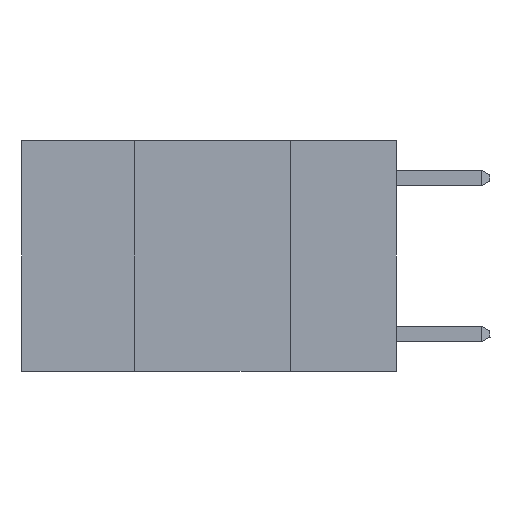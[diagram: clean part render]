
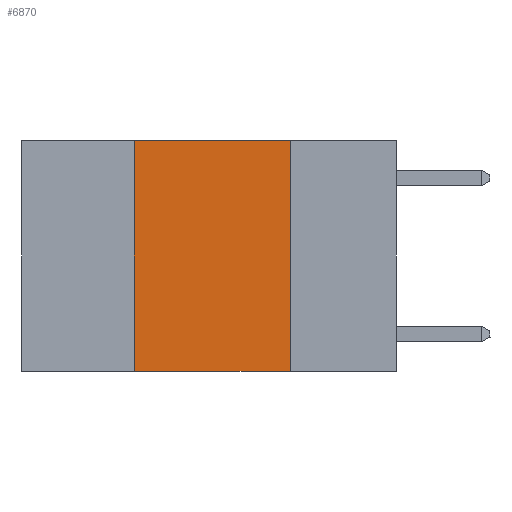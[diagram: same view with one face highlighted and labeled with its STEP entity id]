
A CAD part, left-side view. The second image highlights one B-rep face of the part: STEP entity #6870.
In plain terms, the highlighted planar face has unit normal (-1, 0, 0).
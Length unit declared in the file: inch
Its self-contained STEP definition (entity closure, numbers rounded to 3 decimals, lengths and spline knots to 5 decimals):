
#590 = EDGE_LOOP ( 'NONE', ( #928, #8907, #14900, #12111 ) ) ;
#600 = CARTESIAN_POINT ( 'NONE',  ( 0., 0.42, 0. ) ) ;
#683 = CARTESIAN_POINT ( 'NONE',  ( 0., 0.42, -0.37 ) ) ;
#928 = ORIENTED_EDGE ( 'NONE', *, *, #16280, .F. ) ;
#1712 = LINE ( 'NONE', #1965, #7684 ) ;
#1965 = CARTESIAN_POINT ( 'NONE',  ( 0., 0.17, 0. ) ) ;
#3017 = VECTOR ( 'NONE', #3855, 39.37008 ) ;
#3074 = VECTOR ( 'NONE', #6074, 39.37008 ) ;
#3231 = DIRECTION ( 'NONE',  ( 0., 0., -1. ) ) ;
#3290 = EDGE_CURVE ( 'NONE', #13494, #14641, #10229, .T. ) ;
#3325 = LINE ( 'NONE', #4605, #8217 ) ;
#3855 = DIRECTION ( 'NONE',  ( 0., -1., 0. ) ) ;
#4101 = VERTEX_POINT ( 'NONE', #16416 ) ;
#4605 = CARTESIAN_POINT ( 'NONE',  ( 0., 0.6, -0.37 ) ) ;
#5047 = CARTESIAN_POINT ( 'NONE',  ( 0., 0.6, 0. ) ) ;
#6074 = DIRECTION ( 'NONE',  ( 0., 0., 1. ) ) ;
#6081 = FACE_OUTER_BOUND ( 'NONE', #590, .T. ) ;
#6870 = ADVANCED_FACE ( 'NONE', ( #6081 ), #7169, .F. ) ;
#7169 = PLANE ( 'NONE',  #10882 ) ;
#7684 = VECTOR ( 'NONE', #3231, 39.37008 ) ;
#8217 = VECTOR ( 'NONE', #10784, 39.37008 ) ;
#8272 = CARTESIAN_POINT ( 'NONE',  ( 0., 0.6, 0. ) ) ;
#8687 = CARTESIAN_POINT ( 'NONE',  ( 0., 0.42, 0. ) ) ;
#8907 = ORIENTED_EDGE ( 'NONE', *, *, #3290, .F. ) ;
#10229 = LINE ( 'NONE', #5047, #3017 ) ;
#10784 = DIRECTION ( 'NONE',  ( 0., -1., 0. ) ) ;
#10882 = AXIS2_PLACEMENT_3D ( 'NONE', #8272, #13387, #13465 ) ;
#12111 = ORIENTED_EDGE ( 'NONE', *, *, #14684, .T. ) ;
#13180 = EDGE_CURVE ( 'NONE', #13690, #13494, #14884, .T. ) ;
#13387 = DIRECTION ( 'NONE',  ( 1., 0., 0. ) ) ;
#13465 = DIRECTION ( 'NONE',  ( 0., 0., -1. ) ) ;
#13494 = VERTEX_POINT ( 'NONE', #600 ) ;
#13690 = VERTEX_POINT ( 'NONE', #683 ) ;
#14641 = VERTEX_POINT ( 'NONE', #14736 ) ;
#14684 = EDGE_CURVE ( 'NONE', #13690, #4101, #3325, .T. ) ;
#14736 = CARTESIAN_POINT ( 'NONE',  ( 0., 0.17, 0. ) ) ;
#14884 = LINE ( 'NONE', #8687, #3074 ) ;
#14900 = ORIENTED_EDGE ( 'NONE', *, *, #13180, .F. ) ;
#16280 = EDGE_CURVE ( 'NONE', #14641, #4101, #1712, .T. ) ;
#16416 = CARTESIAN_POINT ( 'NONE',  ( 0., 0.17, -0.37 ) ) ;
